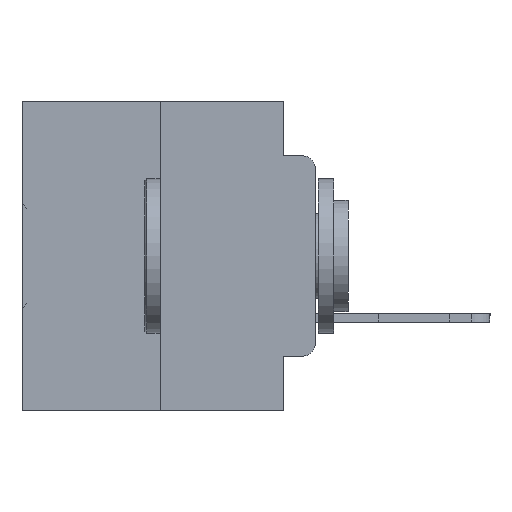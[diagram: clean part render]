
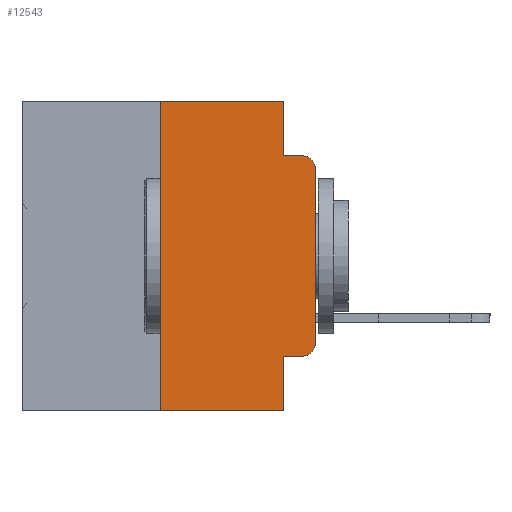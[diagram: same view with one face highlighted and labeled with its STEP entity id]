
A CAD part, left-side view. The second image highlights one B-rep face of the part: STEP entity #12543.
In plain terms, the highlighted planar face has unit normal (-1, 0, 0).
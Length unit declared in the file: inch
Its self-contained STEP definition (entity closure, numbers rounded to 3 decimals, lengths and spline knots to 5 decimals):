
#33 = CARTESIAN_POINT ( 'NONE',  ( 0., 0.051, 0. ) ) ;
#218 = ORIENTED_EDGE ( 'NONE', *, *, #21321, .F. ) ;
#376 = ORIENTED_EDGE ( 'NONE', *, *, #30172, .T. ) ;
#439 = CARTESIAN_POINT ( 'NONE',  ( 0., 0.02, -0.3915 ) ) ;
#495 = FACE_OUTER_BOUND ( 'NONE', #10025, .T. ) ;
#536 = CARTESIAN_POINT ( 'NONE',  ( 0., 0.051, -0.4115 ) ) ;
#598 = DIRECTION ( 'NONE',  ( 0., 0., 1. ) ) ;
#1587 = CARTESIAN_POINT ( 'NONE',  ( 0., 0.25, 0. ) ) ;
#2050 = VECTOR ( 'NONE', #33301, 39.37008 ) ;
#2604 = VECTOR ( 'NONE', #13278, 39.37008 ) ;
#2747 = CARTESIAN_POINT ( 'NONE',  ( 0., 0.051, -0.4115 ) ) ;
#2775 = DIRECTION ( 'NONE',  ( 0., 0., -1. ) ) ;
#2865 = DIRECTION ( 'NONE',  ( 0., 0., -1. ) ) ;
#2903 = LINE ( 'NONE', #7405, #2050 ) ;
#2959 = ORIENTED_EDGE ( 'NONE', *, *, #19324, .T. ) ;
#3005 = AXIS2_PLACEMENT_3D ( 'NONE', #24230, #8393, #26784 ) ;
#3256 = DIRECTION ( 'NONE',  ( 0., 0., -1. ) ) ;
#3558 = VECTOR ( 'NONE', #24351, 39.37008 ) ;
#3985 = DIRECTION ( 'NONE',  ( 0., -1., 0. ) ) ;
#4427 = VERTEX_POINT ( 'NONE', #536 ) ;
#5340 = VERTEX_POINT ( 'NONE', #14521 ) ;
#5864 = CARTESIAN_POINT ( 'NONE',  ( 0., 0.02, -0.1085 ) ) ;
#6558 = ORIENTED_EDGE ( 'NONE', *, *, #14429, .F. ) ;
#6777 = VERTEX_POINT ( 'NONE', #28205 ) ;
#7204 = CIRCLE ( 'NONE', #18150, 0.02 ) ;
#7405 = CARTESIAN_POINT ( 'NONE',  ( 0., 0.473, -0.5 ) ) ;
#7511 = ORIENTED_EDGE ( 'NONE', *, *, #24536, .T. ) ;
#8038 = VECTOR ( 'NONE', #20218, 39.37008 ) ;
#8393 = DIRECTION ( 'NONE',  ( 1., 0., 0. ) ) ;
#8861 = DIRECTION ( 'NONE',  ( 0., 0., -1. ) ) ;
#9104 = CARTESIAN_POINT ( 'NONE',  ( 0., 0.25, 0. ) ) ;
#9561 = CARTESIAN_POINT ( 'NONE',  ( 0., 0.051, -0.0885 ) ) ;
#10025 = EDGE_LOOP ( 'NONE', ( #2959, #22008, #6558, #15861, #21575, #218, #33638, #20499, #376, #7511 ) ) ;
#10163 = VERTEX_POINT ( 'NONE', #19079 ) ;
#10889 = VECTOR ( 'NONE', #2775, 39.37008 ) ;
#11985 = EDGE_CURVE ( 'NONE', #4427, #17004, #14271, .T. ) ;
#12163 = CARTESIAN_POINT ( 'NONE',  ( 0., 0.02, -0.4115 ) ) ;
#12505 = VERTEX_POINT ( 'NONE', #33871 ) ;
#12508 = CARTESIAN_POINT ( 'NONE',  ( 0., 0.051, 0. ) ) ;
#12543 = ADVANCED_FACE ( 'NONE', ( #495 ), #31584, .F. ) ;
#12676 = CARTESIAN_POINT ( 'NONE',  ( 0., 0., -0.3915 ) ) ;
#12892 = VERTEX_POINT ( 'NONE', #12508 ) ;
#13278 = DIRECTION ( 'NONE',  ( 0., 0., 1. ) ) ;
#14271 = LINE ( 'NONE', #31715, #10889 ) ;
#14429 = EDGE_CURVE ( 'NONE', #10163, #12505, #16261, .T. ) ;
#14521 = CARTESIAN_POINT ( 'NONE',  ( 0., 0.25, -0.5 ) ) ;
#15207 = CARTESIAN_POINT ( 'NONE',  ( 0., 0.473, 0. ) ) ;
#15861 = ORIENTED_EDGE ( 'NONE', *, *, #19603, .F. ) ;
#16261 = LINE ( 'NONE', #9561, #8038 ) ;
#16878 = LINE ( 'NONE', #9104, #22002 ) ;
#17004 = VERTEX_POINT ( 'NONE', #23305 ) ;
#17030 = CIRCLE ( 'NONE', #30806, 0.02 ) ;
#17587 = EDGE_CURVE ( 'NONE', #5340, #17004, #2903, .T. ) ;
#18150 = AXIS2_PLACEMENT_3D ( 'NONE', #439, #19688, #3256 ) ;
#19079 = CARTESIAN_POINT ( 'NONE',  ( 0., 0.051, -0.0885 ) ) ;
#19324 = EDGE_CURVE ( 'NONE', #34021, #6777, #22515, .T. ) ;
#19603 = EDGE_CURVE ( 'NONE', #12892, #10163, #22097, .T. ) ;
#19688 = DIRECTION ( 'NONE',  ( -1., 0., 0. ) ) ;
#20218 = DIRECTION ( 'NONE',  ( 0., -1., 0. ) ) ;
#20499 = ORIENTED_EDGE ( 'NONE', *, *, #11985, .F. ) ;
#21321 = EDGE_CURVE ( 'NONE', #5340, #21552, #16878, .T. ) ;
#21552 = VERTEX_POINT ( 'NONE', #1587 ) ;
#21575 = ORIENTED_EDGE ( 'NONE', *, *, #29259, .F. ) ;
#22002 = VECTOR ( 'NONE', #598, 39.37008 ) ;
#22008 = ORIENTED_EDGE ( 'NONE', *, *, #31162, .T. ) ;
#22097 = LINE ( 'NONE', #33, #28882 ) ;
#22515 = LINE ( 'NONE', #28607, #2604 ) ;
#23305 = CARTESIAN_POINT ( 'NONE',  ( 0., 0.051, -0.5 ) ) ;
#23878 = VECTOR ( 'NONE', #3985, 39.37008 ) ;
#24230 = CARTESIAN_POINT ( 'NONE',  ( 0., 0.473, 0. ) ) ;
#24351 = DIRECTION ( 'NONE',  ( 0., -1., 0. ) ) ;
#24536 = EDGE_CURVE ( 'NONE', #29134, #34021, #7204, .T. ) ;
#24639 = DIRECTION ( 'NONE',  ( -1., 0., 0. ) ) ;
#26784 = DIRECTION ( 'NONE',  ( 0., 0., -1. ) ) ;
#28205 = CARTESIAN_POINT ( 'NONE',  ( 0., 0., -0.1085 ) ) ;
#28607 = CARTESIAN_POINT ( 'NONE',  ( 0., 0., 0. ) ) ;
#28882 = VECTOR ( 'NONE', #2865, 39.37008 ) ;
#29134 = VERTEX_POINT ( 'NONE', #12163 ) ;
#29259 = EDGE_CURVE ( 'NONE', #21552, #12892, #31271, .T. ) ;
#30087 = LINE ( 'NONE', #2747, #3558 ) ;
#30172 = EDGE_CURVE ( 'NONE', #4427, #29134, #30087, .T. ) ;
#30806 = AXIS2_PLACEMENT_3D ( 'NONE', #5864, #24639, #8861 ) ;
#31162 = EDGE_CURVE ( 'NONE', #6777, #12505, #17030, .T. ) ;
#31271 = LINE ( 'NONE', #15207, #23878 ) ;
#31584 = PLANE ( 'NONE',  #3005 ) ;
#31715 = CARTESIAN_POINT ( 'NONE',  ( 0., 0.051, 0. ) ) ;
#33301 = DIRECTION ( 'NONE',  ( 0., -1., 0. ) ) ;
#33638 = ORIENTED_EDGE ( 'NONE', *, *, #17587, .T. ) ;
#33871 = CARTESIAN_POINT ( 'NONE',  ( 0., 0.02, -0.0885 ) ) ;
#34021 = VERTEX_POINT ( 'NONE', #12676 ) ;
